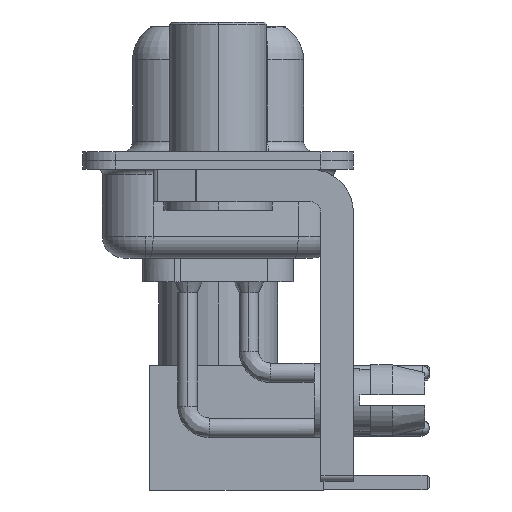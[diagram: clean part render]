
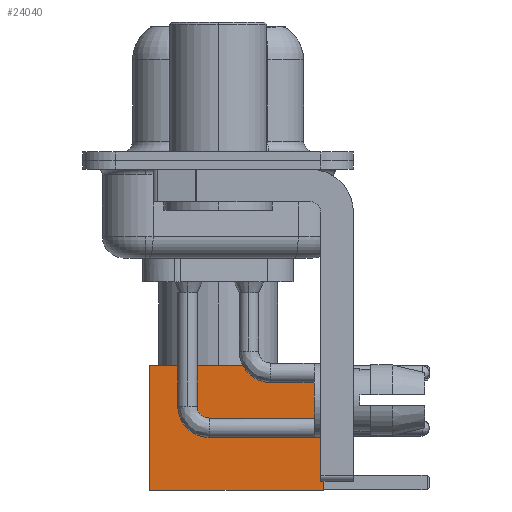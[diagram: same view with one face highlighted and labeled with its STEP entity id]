
A CAD part, left-side view. The second image highlights one B-rep face of the part: STEP entity #24040.
In plain terms, the highlighted face is planar.
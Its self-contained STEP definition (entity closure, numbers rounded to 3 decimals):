
#13 = CARTESIAN_POINT ( 'NONE',  ( -2.875, 2.875, 8. ) ) ;
#1670 = LINE ( 'NONE', #10570, #7169 ) ;
#2390 = CARTESIAN_POINT ( 'NONE',  ( 2.875, 2.875, 0. ) ) ;
#2529 = VECTOR ( 'NONE', #20551, 1000. ) ;
#2583 = ORIENTED_EDGE ( 'NONE', *, *, #10146, .T. ) ;
#4352 = CARTESIAN_POINT ( 'NONE',  ( 2.875, 2.875, 0. ) ) ;
#4522 = DIRECTION ( 'NONE',  ( 0., 1., 0. ) ) ;
#5670 = VECTOR ( 'NONE', #18483, 1000. ) ;
#6404 = EDGE_CURVE ( 'NONE', #8571, #18817, #12929, .T. ) ;
#6423 = DIRECTION ( 'NONE',  ( 0., 0., 1. ) ) ;
#7086 = CARTESIAN_POINT ( 'NONE',  ( 2.875, 2.875, 8. ) ) ;
#7169 = VECTOR ( 'NONE', #18673, 1000. ) ;
#7910 = CARTESIAN_POINT ( 'NONE',  ( 0., 2.875, 8. ) ) ;
#8571 = VERTEX_POINT ( 'NONE', #13 ) ;
#9143 = VERTEX_POINT ( 'NONE', #7086 ) ;
#9479 = EDGE_CURVE ( 'NONE', #9143, #25527, #10521, .T. ) ;
#10146 = EDGE_CURVE ( 'NONE', #25527, #18817, #1670, .T. ) ;
#10521 = LINE ( 'NONE', #4352, #5670 ) ;
#10570 = CARTESIAN_POINT ( 'NONE',  ( 0., 2.875, 0. ) ) ;
#10596 = EDGE_CURVE ( 'NONE', #9143, #8571, #26715, .T. ) ;
#10655 = CARTESIAN_POINT ( 'NONE',  ( -2.875, 2.875, 0. ) ) ;
#12528 = ORIENTED_EDGE ( 'NONE', *, *, #6404, .F. ) ;
#12887 = CARTESIAN_POINT ( 'NONE',  ( 2.875, 2.875, 0. ) ) ;
#12929 = LINE ( 'NONE', #27003, #2529 ) ;
#13605 = AXIS2_PLACEMENT_3D ( 'NONE', #12887, #4522, #6423 ) ;
#14540 = FACE_OUTER_BOUND ( 'NONE', #22305, .T. ) ;
#17737 = ORIENTED_EDGE ( 'NONE', *, *, #9479, .T. ) ;
#18483 = DIRECTION ( 'NONE',  ( 0., 0., -1. ) ) ;
#18673 = DIRECTION ( 'NONE',  ( -1., 0., 0. ) ) ;
#18817 = VERTEX_POINT ( 'NONE', #10655 ) ;
#20412 = DIRECTION ( 'NONE',  ( -1., 0., 0. ) ) ;
#20551 = DIRECTION ( 'NONE',  ( 0., 0., -1. ) ) ;
#22305 = EDGE_LOOP ( 'NONE', ( #17737, #2583, #12528, #24202 ) ) ;
#23887 = VECTOR ( 'NONE', #20412, 1000. ) ;
#24040 = ADVANCED_FACE ( 'NONE', ( #14540 ), #25228, .T. ) ;
#24202 = ORIENTED_EDGE ( 'NONE', *, *, #10596, .F. ) ;
#25228 = PLANE ( 'NONE',  #13605 ) ;
#25527 = VERTEX_POINT ( 'NONE', #2390 ) ;
#26715 = LINE ( 'NONE', #7910, #23887 ) ;
#27003 = CARTESIAN_POINT ( 'NONE',  ( -2.875, 2.875, 0. ) ) ;
